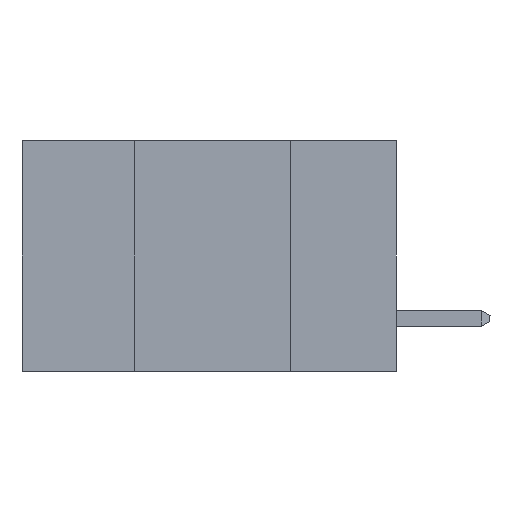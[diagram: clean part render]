
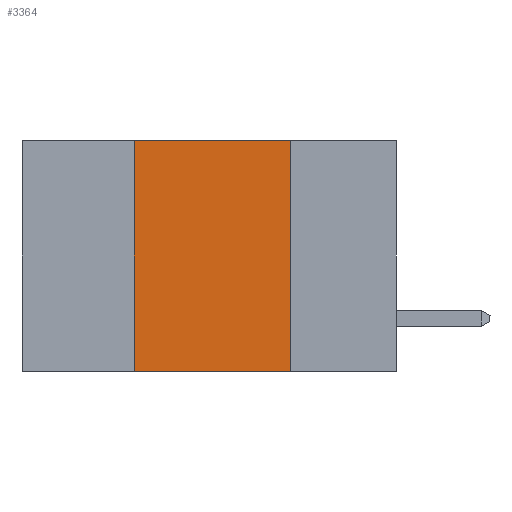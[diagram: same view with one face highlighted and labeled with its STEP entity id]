
A CAD part, left-side view. The second image highlights one B-rep face of the part: STEP entity #3364.
In plain terms, the highlighted planar face has unit normal (-1, 0, 0).
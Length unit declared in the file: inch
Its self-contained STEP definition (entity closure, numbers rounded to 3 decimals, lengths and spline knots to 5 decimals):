
#629 = ORIENTED_EDGE ( 'NONE', *, *, #7475, .F. ) ;
#826 = CARTESIAN_POINT ( 'NONE',  ( 0., 0.42, -0.37 ) ) ;
#1153 = ORIENTED_EDGE ( 'NONE', *, *, #10184, .T. ) ;
#2454 = LINE ( 'NONE', #7138, #9700 ) ;
#2575 = FACE_OUTER_BOUND ( 'NONE', #14099, .T. ) ;
#3190 = DIRECTION ( 'NONE',  ( 0., 0., -1. ) ) ;
#3364 = ADVANCED_FACE ( 'NONE', ( #2575 ), #9379, .F. ) ;
#3614 = CARTESIAN_POINT ( 'NONE',  ( 0., 0.17, 0. ) ) ;
#6413 = VERTEX_POINT ( 'NONE', #18115 ) ;
#6816 = DIRECTION ( 'NONE',  ( 0., 0., 1. ) ) ;
#6844 = CARTESIAN_POINT ( 'NONE',  ( 0., 0.42, -0.37 ) ) ;
#7034 = DIRECTION ( 'NONE',  ( 0., -1., 0. ) ) ;
#7138 = CARTESIAN_POINT ( 'NONE',  ( 0., 0.6, 0. ) ) ;
#7475 = EDGE_CURVE ( 'NONE', #6413, #14321, #2454, .T. ) ;
#7964 = VECTOR ( 'NONE', #9648, 39.37008 ) ;
#8597 = VECTOR ( 'NONE', #6816, 39.37008 ) ;
#9165 = ORIENTED_EDGE ( 'NONE', *, *, #12372, .F. ) ;
#9290 = DIRECTION ( 'NONE',  ( 1., 0., 0. ) ) ;
#9314 = CARTESIAN_POINT ( 'NONE',  ( 0., 0.6, 0. ) ) ;
#9379 = PLANE ( 'NONE',  #13362 ) ;
#9427 = DIRECTION ( 'NONE',  ( 0., 0., -1. ) ) ;
#9568 = CARTESIAN_POINT ( 'NONE',  ( 0., 0.6, -0.37 ) ) ;
#9648 = DIRECTION ( 'NONE',  ( 0., -1., 0. ) ) ;
#9700 = VECTOR ( 'NONE', #7034, 39.37008 ) ;
#10011 = LINE ( 'NONE', #16104, #17073 ) ;
#10184 = EDGE_CURVE ( 'NONE', #16594, #14042, #12280, .T. ) ;
#12280 = LINE ( 'NONE', #9568, #7964 ) ;
#12372 = EDGE_CURVE ( 'NONE', #16594, #6413, #12458, .T. ) ;
#12458 = LINE ( 'NONE', #6844, #8597 ) ;
#13202 = CARTESIAN_POINT ( 'NONE',  ( 0., 0.17, -0.37 ) ) ;
#13362 = AXIS2_PLACEMENT_3D ( 'NONE', #9314, #9290, #9427 ) ;
#14042 = VERTEX_POINT ( 'NONE', #13202 ) ;
#14099 = EDGE_LOOP ( 'NONE', ( #15164, #629, #9165, #1153 ) ) ;
#14321 = VERTEX_POINT ( 'NONE', #3614 ) ;
#15164 = ORIENTED_EDGE ( 'NONE', *, *, #15510, .F. ) ;
#15510 = EDGE_CURVE ( 'NONE', #14321, #14042, #10011, .T. ) ;
#16104 = CARTESIAN_POINT ( 'NONE',  ( 0., 0.17, -0.37 ) ) ;
#16594 = VERTEX_POINT ( 'NONE', #826 ) ;
#17073 = VECTOR ( 'NONE', #3190, 39.37008 ) ;
#18115 = CARTESIAN_POINT ( 'NONE',  ( 0., 0.42, 0. ) ) ;
